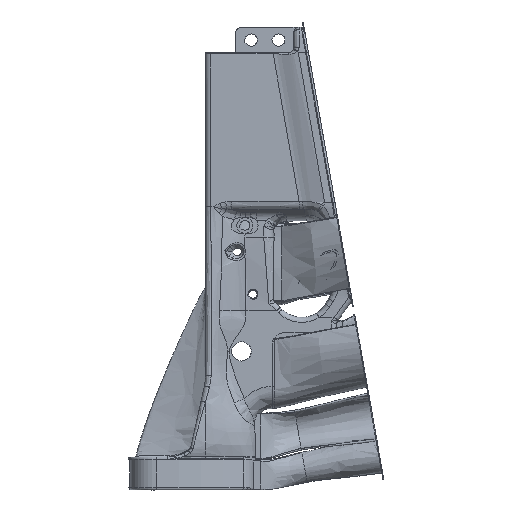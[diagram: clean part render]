
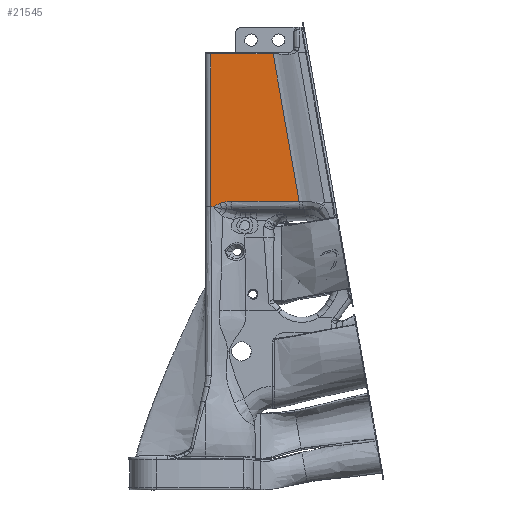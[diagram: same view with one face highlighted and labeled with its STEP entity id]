
A CAD part, left-side view. The second image highlights one B-rep face of the part: STEP entity #21545.
In plain terms, the highlighted planar face has unit normal (-1, 0, 0).
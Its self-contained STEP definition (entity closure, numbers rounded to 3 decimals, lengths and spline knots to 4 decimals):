
#871 = ORIENTED_EDGE ( 'NONE', *, *, #185516, .T. ) ;
#4726 = EDGE_CURVE ( 'NONE', #156601, #76464, #186317, .T. ) ;
#6467 = CARTESIAN_POINT ( 'NONE',  ( -0.78, -0.2494, 3.6478 ) ) ;
#6685 = EDGE_CURVE ( 'NONE', #21032, #207294, #46728, .T. ) ;
#7610 = CARTESIAN_POINT ( 'NONE',  ( -0.78, -0.2574, 3.6526 ) ) ;
#8750 = CARTESIAN_POINT ( 'NONE',  ( -0.78, -0.2239, 3.6331 ) ) ;
#13332 = VECTOR ( 'NONE', #130536, 39.3701 ) ;
#18836 = CARTESIAN_POINT ( 'NONE',  ( -0.78, -0.1, 3.6009 ) ) ;
#21032 = VERTEX_POINT ( 'NONE', #38405 ) ;
#21545 = ADVANCED_FACE ( 'NONE', ( #154445 ), #103153, .T. ) ;
#22803 = CARTESIAN_POINT ( 'NONE',  ( -0.78, -0.2793, 3.6644 ) ) ;
#26005 = EDGE_CURVE ( 'NONE', #201150, #124205, #111053, .T. ) ;
#26300 = CARTESIAN_POINT ( 'NONE',  ( -0.78, -0.3233, 3.679 ) ) ;
#38405 = CARTESIAN_POINT ( 'NONE',  ( -0.78, -1.8484, 3.7058 ) ) ;
#43289 = CARTESIAN_POINT ( 'NONE',  ( -0.78, -0.3956, 3.6953 ) ) ;
#44833 = CARTESIAN_POINT ( 'NONE',  ( -0.78, -0.2051, 3.6234 ) ) ;
#46728 = LINE ( 'NONE', #222621, #171541 ) ;
#49547 = EDGE_LOOP ( 'NONE', ( #177126, #871, #97824, #219534, #194701, #188798, #102901, #191869 ) ) ;
#56263 = EDGE_CURVE ( 'NONE', #76464, #201150, #117302, .T. ) ;
#58883 = CARTESIAN_POINT ( 'NONE',  ( -0.78, -0.225, 3.6338 ) ) ;
#63669 = CARTESIAN_POINT ( 'NONE',  ( -0.78, -0.1, 6.615 ) ) ;
#76464 = VERTEX_POINT ( 'NONE', #160039 ) ;
#77264 = CARTESIAN_POINT ( 'NONE',  ( -0.78, -0.4315, 3.7023 ) ) ;
#77483 = CARTESIAN_POINT ( 'NONE',  ( -0.78, -0.256, 3.6517 ) ) ;
#77692 = CARTESIAN_POINT ( 'NONE',  ( -0.78, -0.5213, 3.7058 ) ) ;
#78265 = B_SPLINE_CURVE_WITH_KNOTS ( 'NONE', 3,
 ( #81213, #134800, #189514, #152270 ),
 .UNSPECIFIED., .F., .F.,
 ( 4, 4 ),
 ( -0.1831, -0.1066 ),
 .UNSPECIFIED. ) ;
#80892 = CARTESIAN_POINT ( 'NONE',  ( -0.78, -0.2262, 3.6344 ) ) ;
#81213 = CARTESIAN_POINT ( 'NONE',  ( -0.78, -0.1, 6.615 ) ) ;
#81275 = CARTESIAN_POINT ( 'NONE',  ( -0.78, -0.1495, 3.6024 ) ) ;
#84718 = CARTESIAN_POINT ( 'NONE',  ( -0.78, -0.1084, 3.6011 ) ) ;
#88099 = EDGE_CURVE ( 'NONE', #129326, #156601, #78265, .T. ) ;
#93799 = CARTESIAN_POINT ( 'NONE',  ( -0.78, -0.2895, 3.6679 ) ) ;
#94438 = LINE ( 'NONE', #125953, #13332 ) ;
#94947 = CARTESIAN_POINT ( 'NONE',  ( -0.78, -0.1638, 3.6064 ) ) ;
#95165 = CARTESIAN_POINT ( 'NONE',  ( -0.78, -0.9637, 3.7058 ) ) ;
#97306 = CARTESIAN_POINT ( 'NONE',  ( -0.78, -0.3587, 3.6881 ) ) ;
#97824 = ORIENTED_EDGE ( 'NONE', *, *, #88099, .T. ) ;
#98365 = CARTESIAN_POINT ( 'NONE',  ( -0.78, -0.269, 3.6595 ) ) ;
#98752 = CARTESIAN_POINT ( 'NONE',  ( -0.78, -0.1, 3.6009 ) ) ;
#99892 = CARTESIAN_POINT ( 'NONE',  ( -0.78, -0.14, 3.6021 ) ) ;
#102901 = ORIENTED_EDGE ( 'NONE', *, *, #184787, .T. ) ;
#103153 = PLANE ( 'NONE',  #205666 ) ;
#103339 = CARTESIAN_POINT ( 'NONE',  ( -0.78, -0.1468, 3.6023 ) ) ;
#105366 = EDGE_CURVE ( 'NONE', #162713, #21032, #211581, .T. ) ;
#111053 = B_SPLINE_CURVE_WITH_KNOTS ( 'NONE', 3,
 ( #225406, #26300, #97306, #199033 ),
 .UNSPECIFIED., .F., .F.,
 ( 4, 4 ),
 ( 0., 1. ),
 .UNSPECIFIED. ) ;
#117302 = B_SPLINE_CURVE_WITH_KNOTS ( 'NONE', 3,
 ( #220737, #94947, #150802, #44833, #219593, #183486, #8750, #58883, #129908, #80892, #184638, #186902, #6467, #167149, #77483, #7610, #98365, #22803, #93799 ),
 .UNSPECIFIED., .F., .F.,
 ( 4, 1, 1, 1, 1, 1, 2, 2, 1, 1, 2, 2, 4 ),
 ( 0., 0.25, 0.375, 0.4375, 0.4687, 0.4844, 0.4922, 0.5, 0.625, 0.6875, 0.7187, 0.75, 1. ),
 .UNSPECIFIED. ) ;
#117395 = CARTESIAN_POINT ( 'NONE',  ( -0.78, -0.1484, 3.6023 ) ) ;
#124205 = VERTEX_POINT ( 'NONE', #43289 ) ;
#125953 = CARTESIAN_POINT ( 'NONE',  ( -0.78, -0.1, 6.615 ) ) ;
#127389 = CARTESIAN_POINT ( 'NONE',  ( -0.78, -0.3956, 3.6953 ) ) ;
#129326 = VERTEX_POINT ( 'NONE', #63669 ) ;
#129908 = CARTESIAN_POINT ( 'NONE',  ( -0.78, -0.2258, 3.6342 ) ) ;
#130536 = DIRECTION ( 'NONE',  ( 0., 1., 0. ) ) ;
#134087 = DIRECTION ( 'NONE',  ( 0., 0.174, 0.985 ) ) ;
#134800 = CARTESIAN_POINT ( 'NONE',  ( -0.78, -0.1, 5.6103 ) ) ;
#148308 = CARTESIAN_POINT ( 'NONE',  ( -0.78, -0.5213, 3.7058 ) ) ;
#150802 = CARTESIAN_POINT ( 'NONE',  ( -0.78, -0.1832, 3.6134 ) ) ;
#152270 = CARTESIAN_POINT ( 'NONE',  ( -0.78, -0.1, 3.6009 ) ) ;
#152332 = CARTESIAN_POINT ( 'NONE',  ( -0.78, -0.1337, 3.6019 ) ) ;
#154445 = FACE_OUTER_BOUND ( 'NONE', #49547, .T. ) ;
#156601 = VERTEX_POINT ( 'NONE', #18836 ) ;
#160039 = CARTESIAN_POINT ( 'NONE',  ( -0.78, -0.1505, 3.6025 ) ) ;
#162713 = VERTEX_POINT ( 'NONE', #210020 ) ;
#163475 = CARTESIAN_POINT ( 'NONE',  ( -0.78, -0.4734, 3.7058 ) ) ;
#166224 = CARTESIAN_POINT ( 'NONE',  ( -0.78, -1.8484, 3.7058 ) ) ;
#167149 = CARTESIAN_POINT ( 'NONE',  ( -0.78, -0.2534, 3.6501 ) ) ;
#169830 = CARTESIAN_POINT ( 'NONE',  ( -0.78, -0.1295, 3.6017 ) ) ;
#170772 = CARTESIAN_POINT ( 'NONE',  ( -0.78, -2.8963, 6.64 ) ) ;
#170969 = CARTESIAN_POINT ( 'NONE',  ( -0.78, -0.15, 3.6023 ) ) ;
#171541 = VECTOR ( 'NONE', #134087, 39.3701 ) ;
#171928 = DIRECTION ( 'NONE',  ( 0., 0., 1. ) ) ;
#177126 = ORIENTED_EDGE ( 'NONE', *, *, #6685, .T. ) ;
#183486 = CARTESIAN_POINT ( 'NONE',  ( -0.78, -0.2212, 3.6317 ) ) ;
#184638 = CARTESIAN_POINT ( 'NONE',  ( -0.78, -0.2319, 3.6377 ) ) ;
#184787 = EDGE_CURVE ( 'NONE', #124205, #162713, #214306, .T. ) ;
#185081 = CARTESIAN_POINT ( 'NONE',  ( -0.78, -0.2895, 3.6679 ) ) ;
#185516 = EDGE_CURVE ( 'NONE', #207294, #129326, #94438, .T. ) ;
#186317 = B_SPLINE_CURVE_WITH_KNOTS ( 'NONE', 3,
 ( #98752, #84718, #190722, #169830, #152332, #99892, #207059, #103339, #117395, #81275, #170969, #223409 ),
 .UNSPECIFIED., .F., .F.,
 ( 4, 2, 2, 1, 1, 2, 4 ),
 ( 0.0024, 0.0031, 0.0034, 0.0035, 0.0036, 0.0037, 0.0037 ),
 .UNSPECIFIED. ) ;
#186902 = CARTESIAN_POINT ( 'NONE',  ( -0.78, -0.24, 3.6423 ) ) ;
#188798 = ORIENTED_EDGE ( 'NONE', *, *, #26005, .T. ) ;
#189514 = CARTESIAN_POINT ( 'NONE',  ( -0.78, -0.1, 4.6056 ) ) ;
#190722 = CARTESIAN_POINT ( 'NONE',  ( -0.78, -0.1168, 3.6014 ) ) ;
#191869 = ORIENTED_EDGE ( 'NONE', *, *, #105366, .T. ) ;
#194701 = ORIENTED_EDGE ( 'NONE', *, *, #56263, .T. ) ;
#199033 = CARTESIAN_POINT ( 'NONE',  ( -0.78, -0.3956, 3.6953 ) ) ;
#201150 = VERTEX_POINT ( 'NONE', #185081 ) ;
#205666 = AXIS2_PLACEMENT_3D ( 'NONE', #170772, #225521, #171928 ) ;
#207059 = CARTESIAN_POINT ( 'NONE',  ( -0.78, -0.1432, 3.6022 ) ) ;
#207294 = VERTEX_POINT ( 'NONE', #220575 ) ;
#210020 = CARTESIAN_POINT ( 'NONE',  ( -0.78, -0.5213, 3.7058 ) ) ;
#211581 = B_SPLINE_CURVE_WITH_KNOTS ( 'NONE', 3,
 ( #77692, #95165, #220946, #166224 ),
 .UNSPECIFIED., .F., .F.,
 ( 4, 4 ),
 ( 0.0266, 0.0603 ),
 .UNSPECIFIED. ) ;
#214306 = B_SPLINE_CURVE_WITH_KNOTS ( 'NONE', 3,
 ( #127389, #77264, #163475, #148308 ),
 .UNSPECIFIED., .F., .F.,
 ( 4, 4 ),
 ( 0., 1. ),
 .UNSPECIFIED. ) ;
#219534 = ORIENTED_EDGE ( 'NONE', *, *, #4726, .T. ) ;
#219593 = CARTESIAN_POINT ( 'NONE',  ( -0.78, -0.2159, 3.6288 ) ) ;
#220575 = CARTESIAN_POINT ( 'NONE',  ( -0.78, -1.3354, 6.615 ) ) ;
#220737 = CARTESIAN_POINT ( 'NONE',  ( -0.78, -0.1505, 3.6025 ) ) ;
#220946 = CARTESIAN_POINT ( 'NONE',  ( -0.78, -1.406, 3.7058 ) ) ;
#222621 = CARTESIAN_POINT ( 'NONE',  ( -0.78, -1.9593, 3.0767 ) ) ;
#223409 = CARTESIAN_POINT ( 'NONE',  ( -0.78, -0.1505, 3.6025 ) ) ;
#225406 = CARTESIAN_POINT ( 'NONE',  ( -0.78, -0.2895, 3.6679 ) ) ;
#225521 = DIRECTION ( 'NONE',  ( -1., 0., 0. ) ) ;
